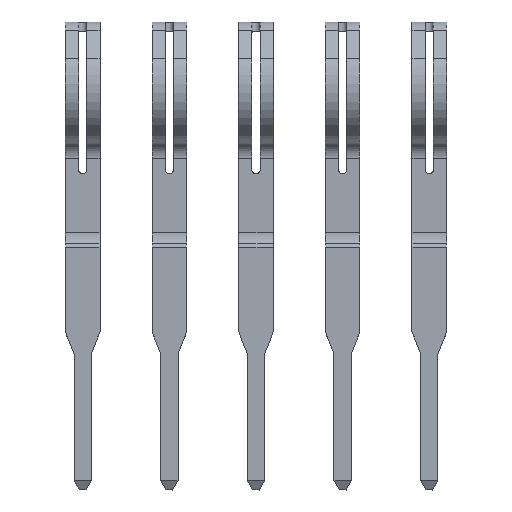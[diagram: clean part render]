
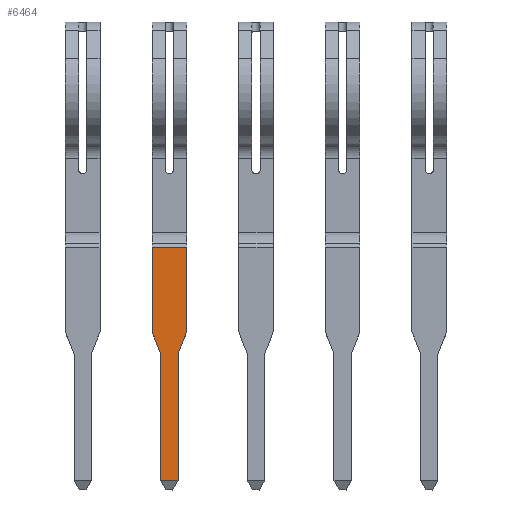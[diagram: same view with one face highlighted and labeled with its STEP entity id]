
A CAD part, top view. The second image highlights one B-rep face of the part: STEP entity #6464.
In plain terms, the highlighted face is planar.
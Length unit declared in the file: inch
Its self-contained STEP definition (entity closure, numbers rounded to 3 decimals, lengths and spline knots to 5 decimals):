
#23 = CARTESIAN_POINT ( 'NONE',  ( 0.60948, 0.0375, 0.01322 ) ) ;
#96 = LINE ( 'NONE', #5033, #269 ) ;
#269 = VECTOR ( 'NONE', #7559, 39.37008 ) ;
#459 = DIRECTION ( 'NONE',  ( -1., 0., 0. ) ) ;
#468 = AXIS2_PLACEMENT_3D ( 'NONE', #4360, #1243, #7965 ) ;
#479 = AXIS2_PLACEMENT_3D ( 'NONE', #2956, #903, #6714 ) ;
#523 = CARTESIAN_POINT ( 'NONE',  ( 0.45821, 0.0375, -0.025 ) ) ;
#571 = DIRECTION ( 'NONE',  ( 1., 0., 0. ) ) ;
#776 = CARTESIAN_POINT ( 'NONE',  ( 0.45821, 0.0375, 0.025 ) ) ;
#798 = DIRECTION ( 'NONE',  ( 1., 0., 0. ) ) ;
#903 = DIRECTION ( 'NONE',  ( 0., -1., 0. ) ) ;
#1209 = EDGE_CURVE ( 'NONE', #7207, #5732, #96, .T. ) ;
#1212 = EDGE_CURVE ( 'NONE', #3609, #3734, #6193, .T. ) ;
#1217 = CARTESIAN_POINT ( 'NONE',  ( 0.45821, 0.0375, -0.025 ) ) ;
#1218 = EDGE_CURVE ( 'NONE', #3734, #1604, #7351, .T. ) ;
#1221 = ORIENTED_EDGE ( 'NONE', *, *, #1252, .T. ) ;
#1225 = EDGE_CURVE ( 'NONE', #1604, #7036, #7840, .T. ) ;
#1227 = EDGE_CURVE ( 'NONE', #7036, #7229, #4029, .T. ) ;
#1239 = EDGE_CURVE ( 'NONE', #7229, #5793, #3766, .T. ) ;
#1242 = EDGE_CURVE ( 'NONE', #5387, #6682, #3957, .T. ) ;
#1243 = DIRECTION ( 'NONE',  ( 0., -1., 0. ) ) ;
#1252 = EDGE_CURVE ( 'NONE', #6682, #3609, #2884, .T. ) ;
#1604 = VERTEX_POINT ( 'NONE', #5282 ) ;
#1654 = ORIENTED_EDGE ( 'NONE', *, *, #4172, .F. ) ;
#1703 = ORIENTED_EDGE ( 'NONE', *, *, #1242, .T. ) ;
#1908 = DIRECTION ( 'NONE',  ( 0., 0., -1. ) ) ;
#1943 = DIRECTION ( 'NONE',  ( 0., -1., 0. ) ) ;
#1963 = CARTESIAN_POINT ( 'NONE',  ( 0.58021, 0.0375, -0.025 ) ) ;
#1987 = CARTESIAN_POINT ( 'NONE',  ( 0.79521, 0.0375, -0.0125 ) ) ;
#2096 = PLANE ( 'NONE',  #3926 ) ;
#2472 = CARTESIAN_POINT ( 'NONE',  ( 0.61321, 0.0375, 0.0125 ) ) ;
#2584 = ORIENTED_EDGE ( 'NONE', *, *, #3601, .F. ) ;
#2761 = DIRECTION ( 'NONE',  ( 0., 0., -1. ) ) ;
#2772 = CARTESIAN_POINT ( 'NONE',  ( 0.58021, 0.0375, -0.025 ) ) ;
#2837 = CARTESIAN_POINT ( 'NONE',  ( 0.45821, 0.0375, 0.025 ) ) ;
#2883 = ORIENTED_EDGE ( 'NONE', *, *, #1209, .T. ) ;
#2884 = CIRCLE ( 'NONE', #468, 0.01 ) ;
#2956 = CARTESIAN_POINT ( 'NONE',  ( 0.61321, 0.0375, -0.0225 ) ) ;
#3601 = EDGE_CURVE ( 'NONE', #7207, #5793, #5765, .T. ) ;
#3609 = VERTEX_POINT ( 'NONE', #8074 ) ;
#3611 = VECTOR ( 'NONE', #6798, 39.37008 ) ;
#3703 = ORIENTED_EDGE ( 'NONE', *, *, #1227, .T. ) ;
#3734 = VERTEX_POINT ( 'NONE', #6748 ) ;
#3758 = ORIENTED_EDGE ( 'NONE', *, *, #1239, .T. ) ;
#3766 = LINE ( 'NONE', #4087, #3611 ) ;
#3926 = AXIS2_PLACEMENT_3D ( 'NONE', #1963, #1943, #1908 ) ;
#3957 = LINE ( 'NONE', #4055, #5061 ) ;
#3986 = VECTOR ( 'NONE', #5919, 39.37008 ) ;
#4029 = CIRCLE ( 'NONE', #479, 0.01 ) ;
#4046 = VECTOR ( 'NONE', #2761, 39.37008 ) ;
#4055 = CARTESIAN_POINT ( 'NONE',  ( 0.58021, 0.0375, 0.025 ) ) ;
#4087 = CARTESIAN_POINT ( 'NONE',  ( 0.58021, 0.0375, -0.025 ) ) ;
#4172 = EDGE_CURVE ( 'NONE', #5387, #5732, #4331, .T. ) ;
#4323 = VECTOR ( 'NONE', #459, 39.37008 ) ;
#4331 = LINE ( 'NONE', #776, #4323 ) ;
#4360 = CARTESIAN_POINT ( 'NONE',  ( 0.61321, 0.0375, 0.0225 ) ) ;
#4496 = FACE_OUTER_BOUND ( 'NONE', #7555, .T. ) ;
#4606 = CARTESIAN_POINT ( 'NONE',  ( 0.61321, 0.0375, -0.0125 ) ) ;
#5033 = CARTESIAN_POINT ( 'NONE',  ( 0.45821, 0.0375, -0.05765 ) ) ;
#5061 = VECTOR ( 'NONE', #7219, 39.37008 ) ;
#5282 = CARTESIAN_POINT ( 'NONE',  ( 0.79521, 0.0375, -0.0125 ) ) ;
#5387 = VERTEX_POINT ( 'NONE', #7172 ) ;
#5732 = VERTEX_POINT ( 'NONE', #2837 ) ;
#5765 = LINE ( 'NONE', #523, #5826 ) ;
#5783 = VECTOR ( 'NONE', #798, 39.37008 ) ;
#5793 = VERTEX_POINT ( 'NONE', #2772 ) ;
#5826 = VECTOR ( 'NONE', #571, 39.37008 ) ;
#5919 = DIRECTION ( 'NONE',  ( -1., 0., 0. ) ) ;
#6193 = LINE ( 'NONE', #2472, #5783 ) ;
#6464 = ADVANCED_FACE ( 'NONE', ( #4496 ), #2096, .F. ) ;
#6682 = VERTEX_POINT ( 'NONE', #23 ) ;
#6714 = DIRECTION ( 'NONE',  ( 1., 0., 0. ) ) ;
#6748 = CARTESIAN_POINT ( 'NONE',  ( 0.79521, 0.0375, 0.0125 ) ) ;
#6798 = DIRECTION ( 'NONE',  ( -0.928, 0., -0.373 ) ) ;
#7036 = VERTEX_POINT ( 'NONE', #7819 ) ;
#7099 = ORIENTED_EDGE ( 'NONE', *, *, #1225, .T. ) ;
#7149 = ORIENTED_EDGE ( 'NONE', *, *, #1218, .T. ) ;
#7172 = CARTESIAN_POINT ( 'NONE',  ( 0.58021, 0.0375, 0.025 ) ) ;
#7207 = VERTEX_POINT ( 'NONE', #1217 ) ;
#7219 = DIRECTION ( 'NONE',  ( 0.928, 0., -0.373 ) ) ;
#7229 = VERTEX_POINT ( 'NONE', #7788 ) ;
#7351 = LINE ( 'NONE', #1987, #4046 ) ;
#7370 = ORIENTED_EDGE ( 'NONE', *, *, #1212, .T. ) ;
#7555 = EDGE_LOOP ( 'NONE', ( #7370, #7149, #7099, #3703, #3758, #2584, #2883, #1654, #1703, #1221 ) ) ;
#7559 = DIRECTION ( 'NONE',  ( 0., 0., 1. ) ) ;
#7788 = CARTESIAN_POINT ( 'NONE',  ( 0.60948, 0.0375, -0.01322 ) ) ;
#7819 = CARTESIAN_POINT ( 'NONE',  ( 0.61321, 0.0375, -0.0125 ) ) ;
#7840 = LINE ( 'NONE', #4606, #3986 ) ;
#7965 = DIRECTION ( 'NONE',  ( -1., 0., 0. ) ) ;
#8074 = CARTESIAN_POINT ( 'NONE',  ( 0.61321, 0.0375, 0.0125 ) ) ;
